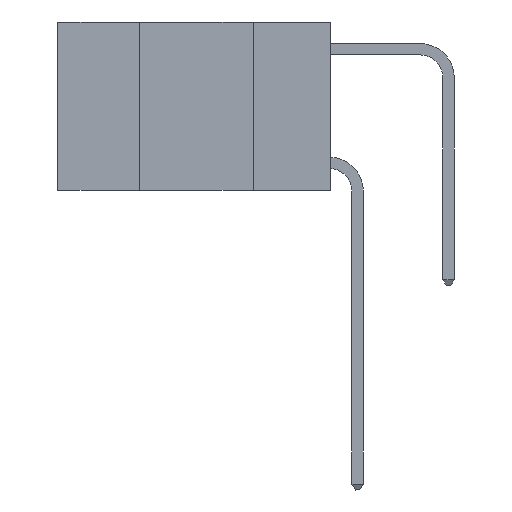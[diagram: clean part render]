
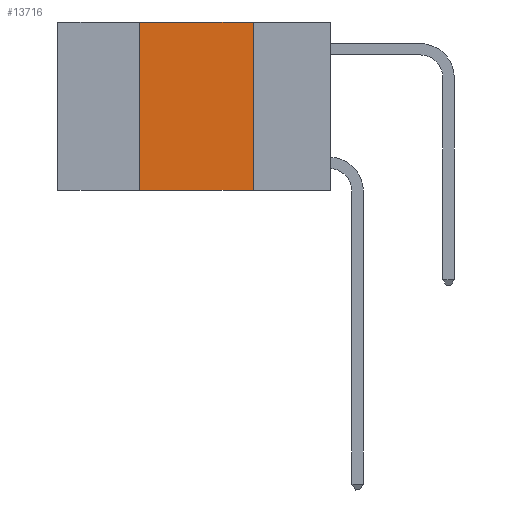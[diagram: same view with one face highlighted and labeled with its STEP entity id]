
A CAD part, left-side view. The second image highlights one B-rep face of the part: STEP entity #13716.
In plain terms, the highlighted planar face has unit normal (-1, 0, 0).
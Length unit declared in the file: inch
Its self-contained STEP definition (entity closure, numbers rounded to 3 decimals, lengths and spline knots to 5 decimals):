
#371 = CARTESIAN_POINT ( 'NONE',  ( 0., 0.42, 0. ) ) ;
#568 = CARTESIAN_POINT ( 'NONE',  ( 0., 0.42, 0. ) ) ;
#585 = EDGE_LOOP ( 'NONE', ( #4185, #9590, #7066, #6672 ) ) ;
#598 = PLANE ( 'NONE',  #4242 ) ;
#1219 = CARTESIAN_POINT ( 'NONE',  ( 0., 0.6, 0. ) ) ;
#2111 = DIRECTION ( 'NONE',  ( 0., -1., 0. ) ) ;
#2422 = VERTEX_POINT ( 'NONE', #568 ) ;
#2665 = VERTEX_POINT ( 'NONE', #9406 ) ;
#4133 = VECTOR ( 'NONE', #13985, 39.37008 ) ;
#4185 = ORIENTED_EDGE ( 'NONE', *, *, #12184, .F. ) ;
#4242 = AXIS2_PLACEMENT_3D ( 'NONE', #9552, #15821, #11972 ) ;
#6337 = CARTESIAN_POINT ( 'NONE',  ( 0., 0.17, 0. ) ) ;
#6437 = LINE ( 'NONE', #371, #16455 ) ;
#6672 = ORIENTED_EDGE ( 'NONE', *, *, #7398, .T. ) ;
#7066 = ORIENTED_EDGE ( 'NONE', *, *, #9327, .F. ) ;
#7398 = EDGE_CURVE ( 'NONE', #15573, #15869, #15537, .T. ) ;
#9327 = EDGE_CURVE ( 'NONE', #15573, #2422, #6437, .T. ) ;
#9406 = CARTESIAN_POINT ( 'NONE',  ( 0., 0.17, 0. ) ) ;
#9552 = CARTESIAN_POINT ( 'NONE',  ( 0., 0.6, 0. ) ) ;
#9590 = ORIENTED_EDGE ( 'NONE', *, *, #13467, .F. ) ;
#9769 = CARTESIAN_POINT ( 'NONE',  ( 0., 0.17, -0.37 ) ) ;
#9942 = LINE ( 'NONE', #6337, #10758 ) ;
#10758 = VECTOR ( 'NONE', #14129, 39.37008 ) ;
#11343 = FACE_OUTER_BOUND ( 'NONE', #585, .T. ) ;
#11972 = DIRECTION ( 'NONE',  ( 0., 0., -1. ) ) ;
#12136 = VECTOR ( 'NONE', #2111, 39.37008 ) ;
#12184 = EDGE_CURVE ( 'NONE', #2665, #15869, #9942, .T. ) ;
#12929 = LINE ( 'NONE', #1219, #4133 ) ;
#13081 = CARTESIAN_POINT ( 'NONE',  ( 0., 0.42, -0.37 ) ) ;
#13467 = EDGE_CURVE ( 'NONE', #2422, #2665, #12929, .T. ) ;
#13716 = ADVANCED_FACE ( 'NONE', ( #11343 ), #598, .F. ) ;
#13985 = DIRECTION ( 'NONE',  ( 0., -1., 0. ) ) ;
#14129 = DIRECTION ( 'NONE',  ( 0., 0., -1. ) ) ;
#14908 = CARTESIAN_POINT ( 'NONE',  ( 0., 0.6, -0.37 ) ) ;
#15537 = LINE ( 'NONE', #14908, #12136 ) ;
#15573 = VERTEX_POINT ( 'NONE', #13081 ) ;
#15821 = DIRECTION ( 'NONE',  ( 1., 0., 0. ) ) ;
#15869 = VERTEX_POINT ( 'NONE', #9769 ) ;
#16071 = DIRECTION ( 'NONE',  ( 0., 0., 1. ) ) ;
#16455 = VECTOR ( 'NONE', #16071, 39.37008 ) ;
